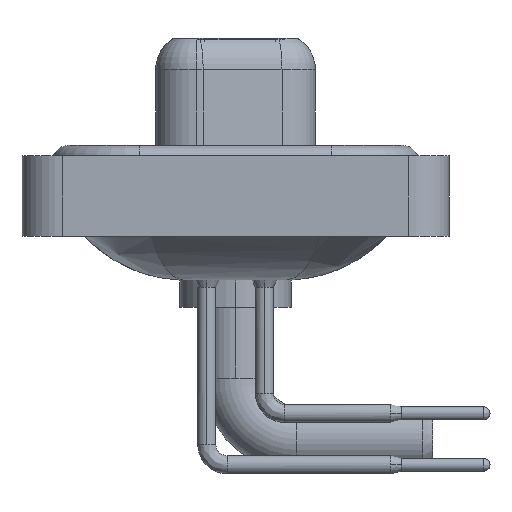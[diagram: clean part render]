
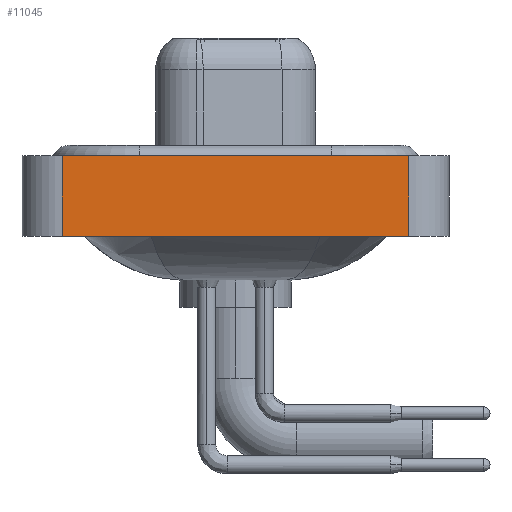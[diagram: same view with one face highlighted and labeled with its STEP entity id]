
A CAD part, left-side view. The second image highlights one B-rep face of the part: STEP entity #11045.
In plain terms, the highlighted planar face has unit normal (-1, 0, 0).
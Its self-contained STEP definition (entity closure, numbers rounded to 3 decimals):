
#93 = EDGE_CURVE ( 'NONE', #13391, #3320, #15182, .T. ) ;
#189 = CARTESIAN_POINT ( 'NONE',  ( -7.3, -8.55, -3.6 ) ) ;
#306 = CARTESIAN_POINT ( 'NONE',  ( -7.3, 8.55, 0.4 ) ) ;
#440 = DIRECTION ( 'NONE',  ( 0., 0., 1. ) ) ;
#1079 = CARTESIAN_POINT ( 'NONE',  ( -7.3, 8.55, -3.6 ) ) ;
#1202 = AXIS2_PLACEMENT_3D ( 'NONE', #17440, #9090, #440 ) ;
#1924 = FACE_OUTER_BOUND ( 'NONE', #19794, .T. ) ;
#2094 = CARTESIAN_POINT ( 'NONE',  ( -7.3, -8.55, -3.6 ) ) ;
#2935 = ORIENTED_EDGE ( 'NONE', *, *, #18697, .F. ) ;
#3320 = VERTEX_POINT ( 'NONE', #7602 ) ;
#4399 = VECTOR ( 'NONE', #17797, 1000. ) ;
#5047 = VERTEX_POINT ( 'NONE', #1079 ) ;
#6468 = ORIENTED_EDGE ( 'NONE', *, *, #93, .F. ) ;
#7294 = EDGE_CURVE ( 'NONE', #9077, #3320, #10942, .T. ) ;
#7602 = CARTESIAN_POINT ( 'NONE',  ( -7.3, -8.55, 0.4 ) ) ;
#8697 = VECTOR ( 'NONE', #11610, 1000. ) ;
#8739 = VECTOR ( 'NONE', #13918, 1000. ) ;
#8764 = PLANE ( 'NONE',  #1202 ) ;
#9077 = VERTEX_POINT ( 'NONE', #21005 ) ;
#9090 = DIRECTION ( 'NONE',  ( -1., 0., 0. ) ) ;
#9160 = LINE ( 'NONE', #16142, #13458 ) ;
#10942 = LINE ( 'NONE', #2094, #4399 ) ;
#11045 = ADVANCED_FACE ( 'NONE', ( #1924 ), #8764, .T. ) ;
#11403 = EDGE_CURVE ( 'NONE', #5047, #9077, #12464, .T. ) ;
#11610 = DIRECTION ( 'NONE',  ( 0., -1., 0. ) ) ;
#12464 = LINE ( 'NONE', #189, #8739 ) ;
#13202 = ORIENTED_EDGE ( 'NONE', *, *, #11403, .T. ) ;
#13391 = VERTEX_POINT ( 'NONE', #306 ) ;
#13458 = VECTOR ( 'NONE', #21437, 1000. ) ;
#13918 = DIRECTION ( 'NONE',  ( 0., -1., 0. ) ) ;
#15182 = LINE ( 'NONE', #22069, #8697 ) ;
#16142 = CARTESIAN_POINT ( 'NONE',  ( -7.3, 8.55, -3.6 ) ) ;
#17440 = CARTESIAN_POINT ( 'NONE',  ( -7.3, -8.55, -3.6 ) ) ;
#17797 = DIRECTION ( 'NONE',  ( 0., 0., 1. ) ) ;
#18124 = ORIENTED_EDGE ( 'NONE', *, *, #7294, .T. ) ;
#18697 = EDGE_CURVE ( 'NONE', #5047, #13391, #9160, .T. ) ;
#19794 = EDGE_LOOP ( 'NONE', ( #18124, #6468, #2935, #13202 ) ) ;
#21005 = CARTESIAN_POINT ( 'NONE',  ( -7.3, -8.55, -3.6 ) ) ;
#21437 = DIRECTION ( 'NONE',  ( 0., 0., 1. ) ) ;
#22069 = CARTESIAN_POINT ( 'NONE',  ( -7.3, -8.55, 0.4 ) ) ;
